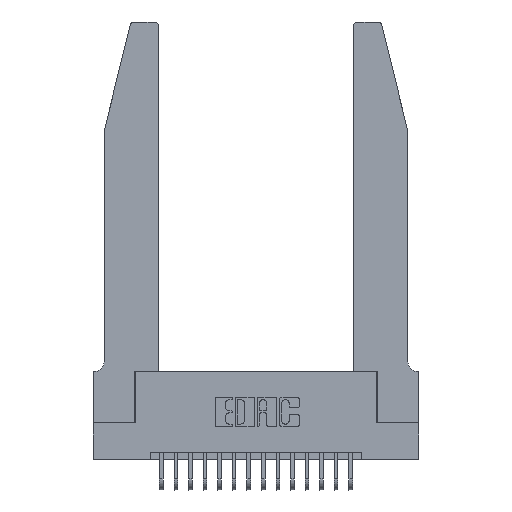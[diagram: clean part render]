
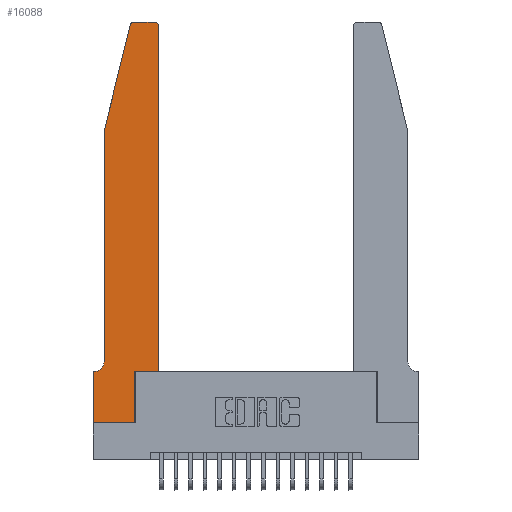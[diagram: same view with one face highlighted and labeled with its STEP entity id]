
A CAD part, top view. The second image highlights one B-rep face of the part: STEP entity #16088.
In plain terms, the highlighted planar face has unit normal (0, 0, 1).
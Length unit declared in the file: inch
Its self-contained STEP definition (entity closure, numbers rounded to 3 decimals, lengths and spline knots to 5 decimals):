
#128 = CARTESIAN_POINT ( 'NONE',  ( 0.2865, 0., 0.37 ) ) ;
#203 = CARTESIAN_POINT ( 'NONE',  ( 0.0755, 2., 0.37 ) ) ;
#342 = DIRECTION ( 'NONE',  ( 1., 0., 0. ) ) ;
#460 = EDGE_CURVE ( 'NONE', #15835, #7168, #649, .T. ) ;
#575 = CARTESIAN_POINT ( 'NONE',  ( 0.2865, 0.35, 0.37 ) ) ;
#649 = CIRCLE ( 'NONE', #12658, 0.03 ) ;
#746 = CARTESIAN_POINT ( 'NONE',  ( 0.0755, 2., 0.37 ) ) ;
#953 = CARTESIAN_POINT ( 'NONE',  ( 0.4505, 0.35, 0.37 ) ) ;
#973 = ORIENTED_EDGE ( 'NONE', *, *, #8461, .T. ) ;
#1058 = CARTESIAN_POINT ( 'NONE',  ( 0.284, 2.72, 0.37 ) ) ;
#1134 = VECTOR ( 'NONE', #10596, 39.37008 ) ;
#2154 = DIRECTION ( 'NONE',  ( 0., -1., 0. ) ) ;
#2210 = LINE ( 'NONE', #2777, #6254 ) ;
#2435 = DIRECTION ( 'NONE',  ( 0., 0., -1. ) ) ;
#2546 = EDGE_CURVE ( 'NONE', #6793, #15835, #10648, .T. ) ;
#2603 = EDGE_LOOP ( 'NONE', ( #5581, #14089, #973, #16225, #19570, #12426, #8811, #20881, #16416, #13079, #17984, #13809 ) ) ;
#2753 = EDGE_CURVE ( 'NONE', #6867, #7566, #8634, .T. ) ;
#2777 = CARTESIAN_POINT ( 'NONE',  ( 0.2865, 0.35, 0.37 ) ) ;
#2823 = DIRECTION ( 'NONE',  ( 1., 0., 0. ) ) ;
#2924 = LINE ( 'NONE', #953, #11295 ) ;
#2933 = EDGE_CURVE ( 'NONE', #12574, #12464, #19794, .T. ) ;
#2973 = CARTESIAN_POINT ( 'NONE',  ( 0.25487, 2.72718, 0.37 ) ) ;
#3206 = LINE ( 'NONE', #8850, #19891 ) ;
#3435 = LINE ( 'NONE', #7508, #20605 ) ;
#3672 = CARTESIAN_POINT ( 'NONE',  ( 0.4205, 2.75, 0.37 ) ) ;
#3800 = VECTOR ( 'NONE', #15179, 39.37008 ) ;
#4522 = DIRECTION ( 'NONE',  ( 1., 0., 0. ) ) ;
#4571 = DIRECTION ( 'NONE',  ( 0., 0., 1. ) ) ;
#4735 = CARTESIAN_POINT ( 'NONE',  ( 0.4205, 2.72, 0.37 ) ) ;
#5581 = ORIENTED_EDGE ( 'NONE', *, *, #13889, .T. ) ;
#6254 = VECTOR ( 'NONE', #18952, 39.37008 ) ;
#6692 = CARTESIAN_POINT ( 'NONE',  ( 0.284, 2.75, 0.37 ) ) ;
#6793 = VERTEX_POINT ( 'NONE', #13957 ) ;
#6867 = VERTEX_POINT ( 'NONE', #18802 ) ;
#6893 = PLANE ( 'NONE',  #10689 ) ;
#7168 = VERTEX_POINT ( 'NONE', #3672 ) ;
#7273 = CARTESIAN_POINT ( 'NONE',  ( 0.2605, 2.75, 0.37 ) ) ;
#7508 = CARTESIAN_POINT ( 'NONE',  ( 0.0755, 2., 0.37 ) ) ;
#7566 = VERTEX_POINT ( 'NONE', #20727 ) ;
#8222 = VERTEX_POINT ( 'NONE', #14542 ) ;
#8276 = LINE ( 'NONE', #203, #3800 ) ;
#8371 = EDGE_CURVE ( 'NONE', #7566, #14703, #13741, .T. ) ;
#8461 = EDGE_CURVE ( 'NONE', #12464, #17306, #3435, .T. ) ;
#8560 = AXIS2_PLACEMENT_3D ( 'NONE', #12416, #2435, #14000 ) ;
#8566 = DIRECTION ( 'NONE',  ( 1., 0., 0. ) ) ;
#8634 = LINE ( 'NONE', #12281, #17599 ) ;
#8748 = AXIS2_PLACEMENT_3D ( 'NONE', #1058, #12765, #2823 ) ;
#8811 = ORIENTED_EDGE ( 'NONE', *, *, #8371, .T. ) ;
#8850 = CARTESIAN_POINT ( 'NONE',  ( 0., 0., 0.37 ) ) ;
#8881 = CARTESIAN_POINT ( 'NONE',  ( 0., 0., 0.37 ) ) ;
#9479 = VECTOR ( 'NONE', #2154, 39.37008 ) ;
#9507 = DIRECTION ( 'NONE',  ( 1., 0., 0. ) ) ;
#9559 = LINE ( 'NONE', #7273, #13817 ) ;
#10264 = EDGE_CURVE ( 'NONE', #8222, #6867, #11498, .T. ) ;
#10596 = DIRECTION ( 'NONE',  ( 0., 1., 0. ) ) ;
#10648 = LINE ( 'NONE', #19622, #1134 ) ;
#10689 = AXIS2_PLACEMENT_3D ( 'NONE', #13361, #18086, #8566 ) ;
#10894 = FACE_OUTER_BOUND ( 'NONE', #2603, .T. ) ;
#11295 = VECTOR ( 'NONE', #9507, 39.37008 ) ;
#11498 = CIRCLE ( 'NONE', #8560, 0.07 ) ;
#12281 = CARTESIAN_POINT ( 'NONE',  ( 0.0755, 0.35, 0.37 ) ) ;
#12416 = CARTESIAN_POINT ( 'NONE',  ( 0.0055, 0.42, 0.37 ) ) ;
#12426 = ORIENTED_EDGE ( 'NONE', *, *, #2753, .T. ) ;
#12464 = VERTEX_POINT ( 'NONE', #2973 ) ;
#12574 = VERTEX_POINT ( 'NONE', #6692 ) ;
#12658 = AXIS2_PLACEMENT_3D ( 'NONE', #4735, #4571, #4522 ) ;
#12765 = DIRECTION ( 'NONE',  ( 0., 0., 1. ) ) ;
#13079 = ORIENTED_EDGE ( 'NONE', *, *, #19977, .T. ) ;
#13361 = CARTESIAN_POINT ( 'NONE',  ( 0., 0.35, 0.37 ) ) ;
#13741 = LINE ( 'NONE', #8881, #9479 ) ;
#13809 = ORIENTED_EDGE ( 'NONE', *, *, #460, .T. ) ;
#13817 = VECTOR ( 'NONE', #20018, 39.37008 ) ;
#13865 = DIRECTION ( 'NONE',  ( -1., 0., 0. ) ) ;
#13889 = EDGE_CURVE ( 'NONE', #7168, #12574, #9559, .T. ) ;
#13957 = CARTESIAN_POINT ( 'NONE',  ( 0.4505, 0.35, 0.37 ) ) ;
#14000 = DIRECTION ( 'NONE',  ( -1., 0., 0. ) ) ;
#14089 = ORIENTED_EDGE ( 'NONE', *, *, #2933, .T. ) ;
#14401 = CARTESIAN_POINT ( 'NONE',  ( 0., 0., 0.37 ) ) ;
#14542 = CARTESIAN_POINT ( 'NONE',  ( 0.0755, 0.42, 0.37 ) ) ;
#14703 = VERTEX_POINT ( 'NONE', #14401 ) ;
#15179 = DIRECTION ( 'NONE',  ( 0., -1., 0. ) ) ;
#15573 = VERTEX_POINT ( 'NONE', #128 ) ;
#15620 = VERTEX_POINT ( 'NONE', #575 ) ;
#15835 = VERTEX_POINT ( 'NONE', #20643 ) ;
#16088 = ADVANCED_FACE ( 'NONE', ( #10894 ), #6893, .T. ) ;
#16225 = ORIENTED_EDGE ( 'NONE', *, *, #17565, .T. ) ;
#16416 = ORIENTED_EDGE ( 'NONE', *, *, #16729, .T. ) ;
#16729 = EDGE_CURVE ( 'NONE', #15573, #15620, #2210, .T. ) ;
#17306 = VERTEX_POINT ( 'NONE', #746 ) ;
#17565 = EDGE_CURVE ( 'NONE', #17306, #8222, #8276, .T. ) ;
#17599 = VECTOR ( 'NONE', #13865, 39.37008 ) ;
#17984 = ORIENTED_EDGE ( 'NONE', *, *, #2546, .T. ) ;
#18086 = DIRECTION ( 'NONE',  ( 0., 0., 1. ) ) ;
#18640 = DIRECTION ( 'NONE',  ( -0.239, -0.971, 0. ) ) ;
#18802 = CARTESIAN_POINT ( 'NONE',  ( 0.0055, 0.35, 0.37 ) ) ;
#18952 = DIRECTION ( 'NONE',  ( 0., 1., 0. ) ) ;
#19570 = ORIENTED_EDGE ( 'NONE', *, *, #10264, .T. ) ;
#19622 = CARTESIAN_POINT ( 'NONE',  ( 0.4505, 0.35, 0.37 ) ) ;
#19754 = EDGE_CURVE ( 'NONE', #14703, #15573, #3206, .T. ) ;
#19794 = CIRCLE ( 'NONE', #8748, 0.03 ) ;
#19891 = VECTOR ( 'NONE', #342, 39.37008 ) ;
#19977 = EDGE_CURVE ( 'NONE', #15620, #6793, #2924, .T. ) ;
#20018 = DIRECTION ( 'NONE',  ( -1., 0., 0. ) ) ;
#20605 = VECTOR ( 'NONE', #18640, 39.37008 ) ;
#20643 = CARTESIAN_POINT ( 'NONE',  ( 0.4505, 2.72, 0.37 ) ) ;
#20727 = CARTESIAN_POINT ( 'NONE',  ( 0., 0.35, 0.37 ) ) ;
#20881 = ORIENTED_EDGE ( 'NONE', *, *, #19754, .T. ) ;
